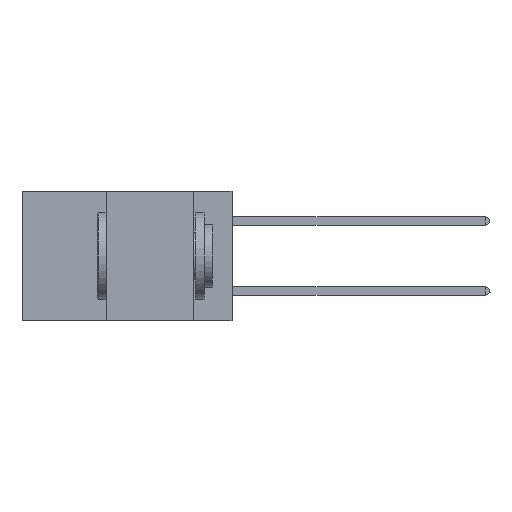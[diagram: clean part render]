
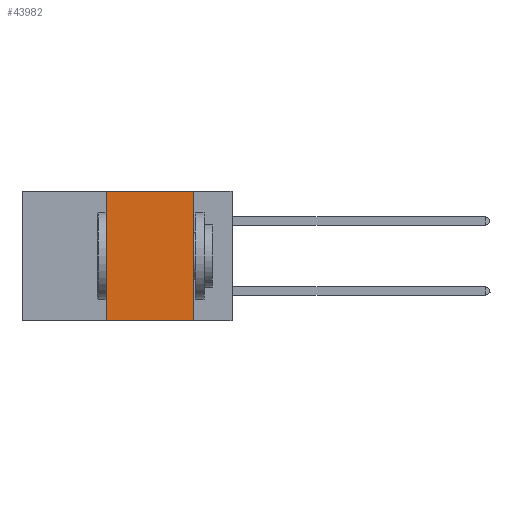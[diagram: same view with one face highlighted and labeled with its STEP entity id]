
A CAD part, left-side view. The second image highlights one B-rep face of the part: STEP entity #43982.
In plain terms, the highlighted planar face has unit normal (-1, 0, 0).
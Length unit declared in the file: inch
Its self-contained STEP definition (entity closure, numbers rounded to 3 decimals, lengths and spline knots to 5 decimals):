
#2289 = CARTESIAN_POINT ( 'NONE',  ( 0., 0.11, 0. ) ) ;
#2786 = VECTOR ( 'NONE', #4207, 39.37008 ) ;
#4207 = DIRECTION ( 'NONE',  ( 0., -1., 0. ) ) ;
#5879 = VERTEX_POINT ( 'NONE', #41114 ) ;
#6055 = DIRECTION ( 'NONE',  ( 0., 0., -1. ) ) ;
#9531 = ORIENTED_EDGE ( 'NONE', *, *, #19561, .T. ) ;
#10061 = AXIS2_PLACEMENT_3D ( 'NONE', #13718, #41551, #20677 ) ;
#10161 = CARTESIAN_POINT ( 'NONE',  ( 0., 0.6, -0.37 ) ) ;
#10668 = EDGE_CURVE ( 'NONE', #43807, #15980, #25752, .T. ) ;
#11343 = ORIENTED_EDGE ( 'NONE', *, *, #17431, .F. ) ;
#13718 = CARTESIAN_POINT ( 'NONE',  ( 0., 0.6, 0. ) ) ;
#13907 = EDGE_LOOP ( 'NONE', ( #30489, #11343, #29027, #9531 ) ) ;
#15980 = VERTEX_POINT ( 'NONE', #42477 ) ;
#17431 = EDGE_CURVE ( 'NONE', #5879, #43807, #40699, .T. ) ;
#18733 = VECTOR ( 'NONE', #40301, 39.37008 ) ;
#19561 = EDGE_CURVE ( 'NONE', #43840, #15980, #29724, .T. ) ;
#20677 = DIRECTION ( 'NONE',  ( 0., 0., -1. ) ) ;
#22156 = EDGE_CURVE ( 'NONE', #43840, #5879, #31710, .T. ) ;
#24772 = DIRECTION ( 'NONE',  ( 0., 0., 1. ) ) ;
#25752 = LINE ( 'NONE', #37338, #37783 ) ;
#28023 = PLANE ( 'NONE',  #10061 ) ;
#29027 = ORIENTED_EDGE ( 'NONE', *, *, #22156, .F. ) ;
#29724 = LINE ( 'NONE', #10161, #2786 ) ;
#30489 = ORIENTED_EDGE ( 'NONE', *, *, #10668, .F. ) ;
#30794 = CARTESIAN_POINT ( 'NONE',  ( 0., 0.36, -0.37 ) ) ;
#31710 = LINE ( 'NONE', #31766, #42739 ) ;
#31766 = CARTESIAN_POINT ( 'NONE',  ( 0., 0.36, 0. ) ) ;
#37338 = CARTESIAN_POINT ( 'NONE',  ( 0., 0.11, 0. ) ) ;
#37783 = VECTOR ( 'NONE', #6055, 39.37008 ) ;
#40301 = DIRECTION ( 'NONE',  ( 0., -1., 0. ) ) ;
#40699 = LINE ( 'NONE', #43828, #18733 ) ;
#41114 = CARTESIAN_POINT ( 'NONE',  ( 0., 0.36, 0. ) ) ;
#41551 = DIRECTION ( 'NONE',  ( 1., 0., 0. ) ) ;
#41851 = FACE_OUTER_BOUND ( 'NONE', #13907, .T. ) ;
#42477 = CARTESIAN_POINT ( 'NONE',  ( 0., 0.11, -0.37 ) ) ;
#42739 = VECTOR ( 'NONE', #24772, 39.37008 ) ;
#43807 = VERTEX_POINT ( 'NONE', #2289 ) ;
#43828 = CARTESIAN_POINT ( 'NONE',  ( 0., 0.6, 0. ) ) ;
#43840 = VERTEX_POINT ( 'NONE', #30794 ) ;
#43982 = ADVANCED_FACE ( 'NONE', ( #41851 ), #28023, .F. ) ;
